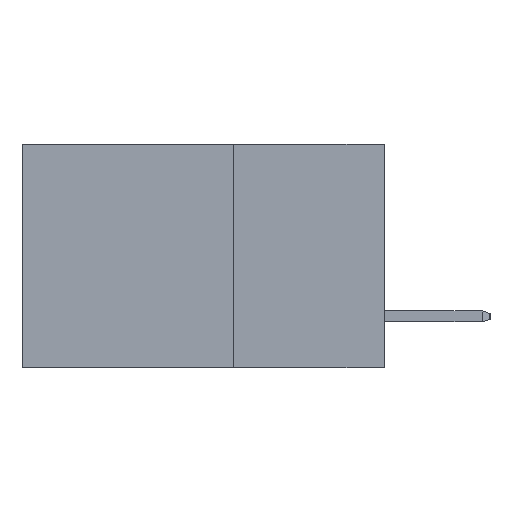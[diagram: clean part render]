
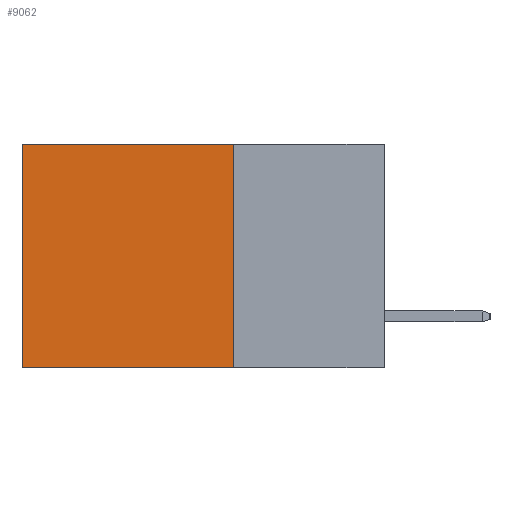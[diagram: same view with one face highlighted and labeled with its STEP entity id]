
A CAD part, left-side view. The second image highlights one B-rep face of the part: STEP entity #9062.
In plain terms, the highlighted planar face has unit normal (-1, 0, 0).
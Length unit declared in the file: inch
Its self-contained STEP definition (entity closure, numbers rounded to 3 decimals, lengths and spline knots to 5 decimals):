
#11 = DIRECTION ( 'NONE',  ( 0., 0., -1. ) ) ;
#941 = VECTOR ( 'NONE', #17941, 39.37008 ) ;
#972 = CARTESIAN_POINT ( 'NONE',  ( 0.298, 0.25, -0.37 ) ) ;
#4729 = CARTESIAN_POINT ( 'NONE',  ( 0.298, 0.25, 0. ) ) ;
#5002 = CARTESIAN_POINT ( 'NONE',  ( 0.298, 0.25, 0. ) ) ;
#5377 = LINE ( 'NONE', #4729, #941 ) ;
#5889 = VECTOR ( 'NONE', #20280, 39.37008 ) ;
#5930 = LINE ( 'NONE', #972, #13727 ) ;
#6618 = EDGE_LOOP ( 'NONE', ( #11820, #7944, #17442, #16526 ) ) ;
#6664 = VECTOR ( 'NONE', #15703, 39.37008 ) ;
#7944 = ORIENTED_EDGE ( 'NONE', *, *, #16668, .F. ) ;
#8337 = PLANE ( 'NONE',  #16068 ) ;
#8417 = VERTEX_POINT ( 'NONE', #16642 ) ;
#9062 = ADVANCED_FACE ( 'NONE', ( #16385 ), #8337, .F. ) ;
#10024 = DIRECTION ( 'NONE',  ( 1., 0., 0. ) ) ;
#10940 = DIRECTION ( 'NONE',  ( 0., 1., 0. ) ) ;
#10984 = EDGE_CURVE ( 'NONE', #13932, #20143, #5377, .T. ) ;
#11127 = CARTESIAN_POINT ( 'NONE',  ( 0.298, 0.6, 0. ) ) ;
#11820 = ORIENTED_EDGE ( 'NONE', *, *, #19330, .T. ) ;
#13727 = VECTOR ( 'NONE', #10940, 39.37008 ) ;
#13932 = VERTEX_POINT ( 'NONE', #19283 ) ;
#14073 = CARTESIAN_POINT ( 'NONE',  ( 0.298, 0.6, 0. ) ) ;
#15451 = LINE ( 'NONE', #14073, #6664 ) ;
#15630 = VERTEX_POINT ( 'NONE', #11127 ) ;
#15703 = DIRECTION ( 'NONE',  ( 0., 0., -1. ) ) ;
#16068 = AXIS2_PLACEMENT_3D ( 'NONE', #5002, #10024, #11 ) ;
#16108 = CARTESIAN_POINT ( 'NONE',  ( 0.298, 0.25, -0.37 ) ) ;
#16385 = FACE_OUTER_BOUND ( 'NONE', #6618, .T. ) ;
#16526 = ORIENTED_EDGE ( 'NONE', *, *, #19207, .T. ) ;
#16642 = CARTESIAN_POINT ( 'NONE',  ( 0.298, 0.6, -0.37 ) ) ;
#16668 = EDGE_CURVE ( 'NONE', #20143, #8417, #5930, .T. ) ;
#17442 = ORIENTED_EDGE ( 'NONE', *, *, #10984, .F. ) ;
#17941 = DIRECTION ( 'NONE',  ( 0., 0., -1. ) ) ;
#18530 = LINE ( 'NONE', #18636, #5889 ) ;
#18636 = CARTESIAN_POINT ( 'NONE',  ( 0.298, 0.25, 0. ) ) ;
#19207 = EDGE_CURVE ( 'NONE', #13932, #15630, #18530, .T. ) ;
#19283 = CARTESIAN_POINT ( 'NONE',  ( 0.298, 0.25, 0. ) ) ;
#19330 = EDGE_CURVE ( 'NONE', #15630, #8417, #15451, .T. ) ;
#20143 = VERTEX_POINT ( 'NONE', #16108 ) ;
#20280 = DIRECTION ( 'NONE',  ( 0., 1., 0. ) ) ;
